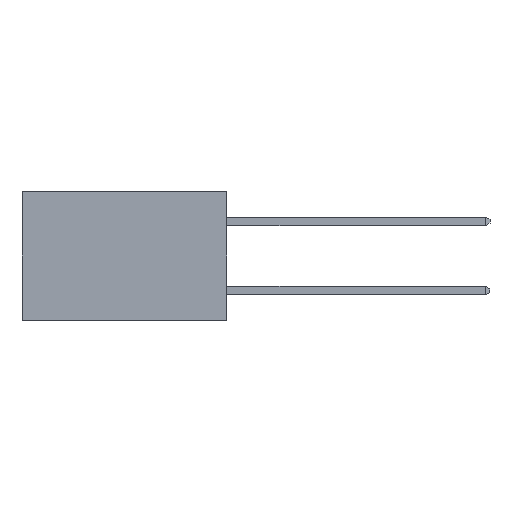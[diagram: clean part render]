
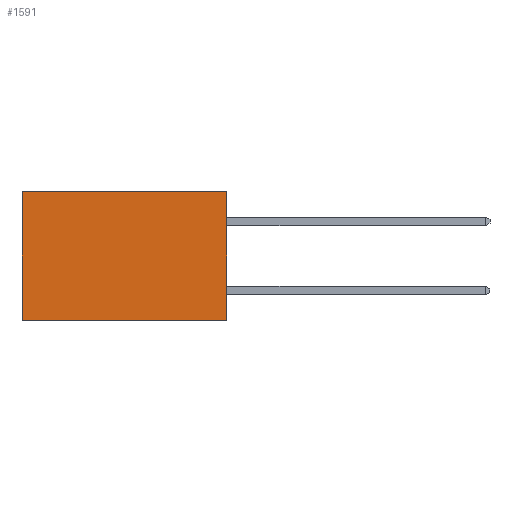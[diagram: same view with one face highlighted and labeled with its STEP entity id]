
A CAD part, left-side view. The second image highlights one B-rep face of the part: STEP entity #1591.
In plain terms, the highlighted planar face has unit normal (-1, 0, 0).
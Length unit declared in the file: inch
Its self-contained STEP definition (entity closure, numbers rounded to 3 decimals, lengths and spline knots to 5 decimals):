
#389 = VERTEX_POINT ( 'NONE', #2286 ) ;
#511 = LINE ( 'NONE', #4823, #6369 ) ;
#1113 = ORIENTED_EDGE ( 'NONE', *, *, #2128, .F. ) ;
#1140 = ORIENTED_EDGE ( 'NONE', *, *, #2715, .T. ) ;
#1229 = EDGE_CURVE ( 'NONE', #1741, #389, #5933, .T. ) ;
#1454 = CARTESIAN_POINT ( 'NONE',  ( 0.277, 0., -0.37 ) ) ;
#1573 = CARTESIAN_POINT ( 'NONE',  ( 0.277, 0., 0. ) ) ;
#1591 = ADVANCED_FACE ( 'NONE', ( #6311 ), #3936, .F. ) ;
#1678 = LINE ( 'NONE', #3085, #4776 ) ;
#1688 = VERTEX_POINT ( 'NONE', #4627 ) ;
#1741 = VERTEX_POINT ( 'NONE', #1573 ) ;
#1776 = ORIENTED_EDGE ( 'NONE', *, *, #2329, .F. ) ;
#2128 = EDGE_CURVE ( 'NONE', #1741, #1688, #1678, .T. ) ;
#2286 = CARTESIAN_POINT ( 'NONE',  ( 0.277, 0.59, 0. ) ) ;
#2329 = EDGE_CURVE ( 'NONE', #1688, #6188, #511, .T. ) ;
#2427 = LINE ( 'NONE', #7147, #3761 ) ;
#2715 = EDGE_CURVE ( 'NONE', #389, #6188, #2427, .T. ) ;
#2727 = ORIENTED_EDGE ( 'NONE', *, *, #1229, .T. ) ;
#2943 = EDGE_LOOP ( 'NONE', ( #1140, #1776, #1113, #2727 ) ) ;
#3083 = DIRECTION ( 'NONE',  ( 0., 0., -1. ) ) ;
#3085 = CARTESIAN_POINT ( 'NONE',  ( 0.277, 0., -0.37 ) ) ;
#3554 = DIRECTION ( 'NONE',  ( 0., 0., -1. ) ) ;
#3761 = VECTOR ( 'NONE', #6809, 39.37008 ) ;
#3936 = PLANE ( 'NONE',  #5741 ) ;
#4627 = CARTESIAN_POINT ( 'NONE',  ( 0.277, 0., -0.37 ) ) ;
#4648 = VECTOR ( 'NONE', #5032, 39.37008 ) ;
#4707 = CARTESIAN_POINT ( 'NONE',  ( 0.277, 0., 0. ) ) ;
#4776 = VECTOR ( 'NONE', #3083, 39.37008 ) ;
#4823 = CARTESIAN_POINT ( 'NONE',  ( 0.277, 0., -0.37 ) ) ;
#5031 = DIRECTION ( 'NONE',  ( 0., 1., 0. ) ) ;
#5032 = DIRECTION ( 'NONE',  ( 0., 1., 0. ) ) ;
#5273 = DIRECTION ( 'NONE',  ( 1., 0., 0. ) ) ;
#5741 = AXIS2_PLACEMENT_3D ( 'NONE', #1454, #5273, #3554 ) ;
#5933 = LINE ( 'NONE', #4707, #4648 ) ;
#6188 = VERTEX_POINT ( 'NONE', #7016 ) ;
#6311 = FACE_OUTER_BOUND ( 'NONE', #2943, .T. ) ;
#6369 = VECTOR ( 'NONE', #5031, 39.37008 ) ;
#6809 = DIRECTION ( 'NONE',  ( 0., 0., -1. ) ) ;
#7016 = CARTESIAN_POINT ( 'NONE',  ( 0.277, 0.59, -0.37 ) ) ;
#7147 = CARTESIAN_POINT ( 'NONE',  ( 0.277, 0.59, -0.37 ) ) ;
